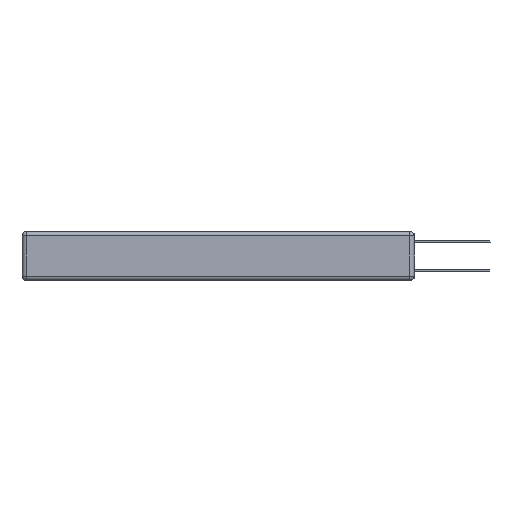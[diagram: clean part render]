
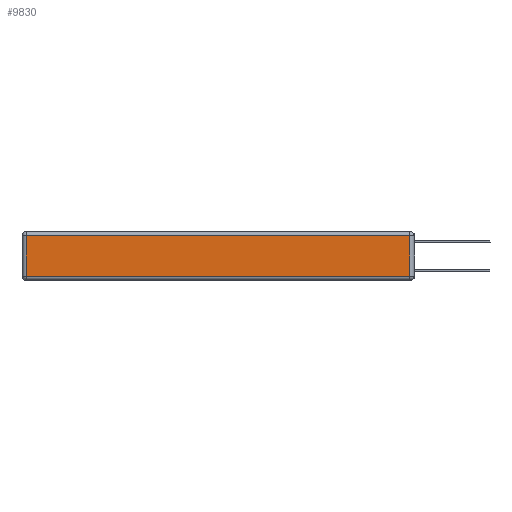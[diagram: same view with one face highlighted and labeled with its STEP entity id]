
A CAD part, left-side view. The second image highlights one B-rep face of the part: STEP entity #9830.
In plain terms, the highlighted planar face has unit normal (-1, 0, 0).
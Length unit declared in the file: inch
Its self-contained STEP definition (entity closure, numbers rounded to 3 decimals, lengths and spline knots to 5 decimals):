
#588 = LINE ( 'NONE', #6082, #2699 ) ;
#1122 = EDGE_CURVE ( 'NONE', #14374, #6967, #9269, .T. ) ;
#1572 = VECTOR ( 'NONE', #14539, 39.37008 ) ;
#1786 = LINE ( 'NONE', #7795, #1572 ) ;
#2073 = DIRECTION ( 'NONE',  ( -1., 0., 0. ) ) ;
#2152 = CARTESIAN_POINT ( 'NONE',  ( 0., 2.72, -0.313 ) ) ;
#2198 = DIRECTION ( 'NONE',  ( 0., 0., -1. ) ) ;
#2699 = VECTOR ( 'NONE', #14094, 39.37008 ) ;
#2830 = ORIENTED_EDGE ( 'NONE', *, *, #1122, .T. ) ;
#2868 = CARTESIAN_POINT ( 'NONE',  ( 0., 0.03, -0.313 ) ) ;
#3177 = EDGE_CURVE ( 'NONE', #6967, #4400, #7726, .T. ) ;
#3917 = ORIENTED_EDGE ( 'NONE', *, *, #4867, .T. ) ;
#4313 = FACE_OUTER_BOUND ( 'NONE', #9503, .T. ) ;
#4400 = VERTEX_POINT ( 'NONE', #2868 ) ;
#4867 = EDGE_CURVE ( 'NONE', #4400, #5333, #588, .T. ) ;
#5058 = EDGE_CURVE ( 'NONE', #5333, #14374, #1786, .T. ) ;
#5246 = DIRECTION ( 'NONE',  ( 0., -1., 0. ) ) ;
#5333 = VERTEX_POINT ( 'NONE', #9596 ) ;
#6082 = CARTESIAN_POINT ( 'NONE',  ( 0., 0.03, -0.343 ) ) ;
#6587 = DIRECTION ( 'NONE',  ( 0., 0., 1. ) ) ;
#6813 = CARTESIAN_POINT ( 'NONE',  ( 0., 2.72, -0.03 ) ) ;
#6967 = VERTEX_POINT ( 'NONE', #2152 ) ;
#7297 = VECTOR ( 'NONE', #5246, 39.37008 ) ;
#7726 = LINE ( 'NONE', #14474, #7297 ) ;
#7795 = CARTESIAN_POINT ( 'NONE',  ( 0., 2.75, -0.03 ) ) ;
#8134 = CARTESIAN_POINT ( 'NONE',  ( 0., 2.72, -0.343 ) ) ;
#8367 = ORIENTED_EDGE ( 'NONE', *, *, #5058, .T. ) ;
#9269 = LINE ( 'NONE', #8134, #14823 ) ;
#9503 = EDGE_LOOP ( 'NONE', ( #12902, #3917, #8367, #2830 ) ) ;
#9596 = CARTESIAN_POINT ( 'NONE',  ( 0., 0.03, -0.03 ) ) ;
#9830 = ADVANCED_FACE ( 'NONE', ( #4313 ), #13236, .T. ) ;
#12273 = CARTESIAN_POINT ( 'NONE',  ( 0., 0., -0.343 ) ) ;
#12749 = AXIS2_PLACEMENT_3D ( 'NONE', #12273, #2073, #6587 ) ;
#12902 = ORIENTED_EDGE ( 'NONE', *, *, #3177, .T. ) ;
#13236 = PLANE ( 'NONE',  #12749 ) ;
#14094 = DIRECTION ( 'NONE',  ( 0., 0., 1. ) ) ;
#14374 = VERTEX_POINT ( 'NONE', #6813 ) ;
#14474 = CARTESIAN_POINT ( 'NONE',  ( 0., 0., -0.313 ) ) ;
#14539 = DIRECTION ( 'NONE',  ( 0., 1., 0. ) ) ;
#14823 = VECTOR ( 'NONE', #2198, 39.37008 ) ;
